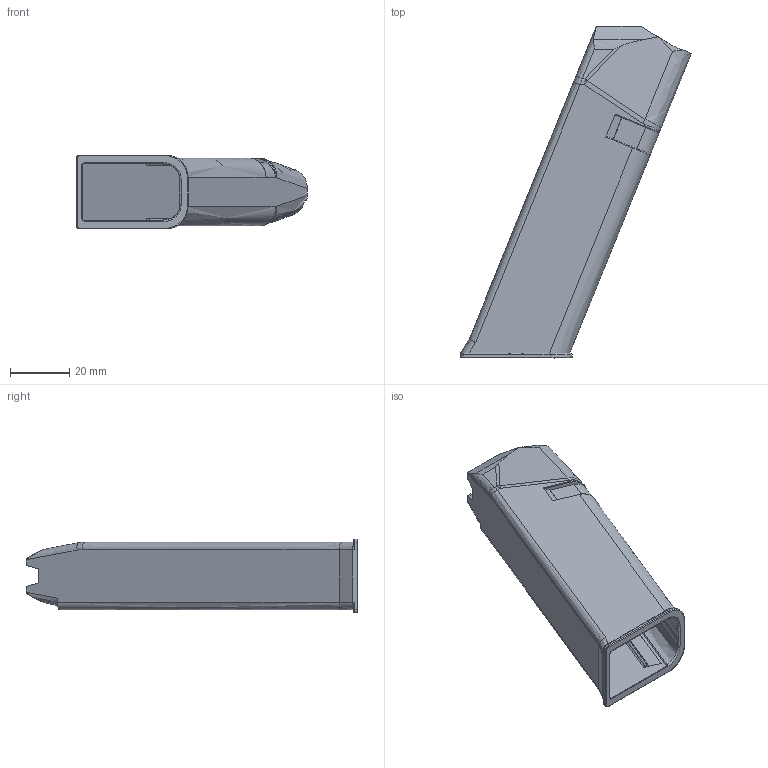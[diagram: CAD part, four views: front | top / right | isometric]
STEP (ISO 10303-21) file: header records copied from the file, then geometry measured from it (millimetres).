
FILE_DESCRIPTION(/* description */ (''),/* implementation_level */ '2;1');
FILE_NAME(/* name *//* time_stamp *//* author */ (''),/* organization */ (''),/* preprocessor_version */ 'ST-DEVELOPER v18.1',/* originating_system */ 'Autodesk Translation Framework v9.3.0.1241',/* authorisation */ '');
FILE_SCHEMA (('AUTOMOTIVE_DESIGN { 1 0 10303 214 3 1 1 }'));
Length unit declared in the file: millimetre
Products named in the file (1): Menendez Mag Body V1.61
Bounding box: 77.74 x 111.88 x 24.87 mm (x, y, z)
Volume: 20184.3 mm3; surface area: 23889 mm2
Topology: 1 solids, 5 shells, 400 faces, 1059 edges, 662 vertices
Faces by surface type: plane 228, bspline 134, cylinder 36, cone 2
Entity records: 15048 total; most frequent: CARTESIAN_POINT 5746, ORIENTED_EDGE 2108, DIRECTION 1686, EDGE_CURVE 1054, LINE 666, VECTOR 666, VERTEX_POINT 662, AXIS2_PLACEMENT_3D 510
